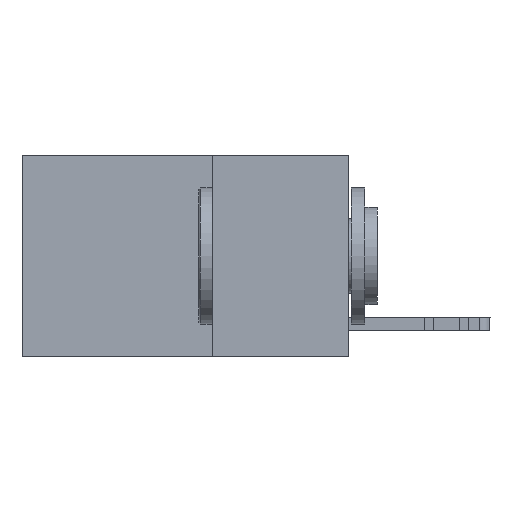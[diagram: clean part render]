
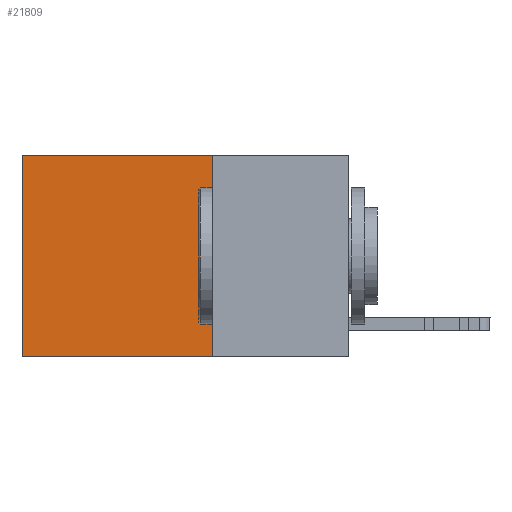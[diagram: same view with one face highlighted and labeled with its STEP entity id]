
A CAD part, left-side view. The second image highlights one B-rep face of the part: STEP entity #21809.
In plain terms, the highlighted planar face has unit normal (-1, 0, 0).
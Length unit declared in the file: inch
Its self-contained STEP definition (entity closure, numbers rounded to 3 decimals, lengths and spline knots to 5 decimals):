
#1019 = DIRECTION ( 'NONE',  ( 0., 0., -1. ) ) ;
#2023 = EDGE_CURVE ( 'NONE', #22591, #15932, #2679, .T. ) ;
#2591 = EDGE_CURVE ( 'NONE', #4354, #22591, #20277, .T. ) ;
#2679 = LINE ( 'NONE', #14874, #13444 ) ;
#3174 = VECTOR ( 'NONE', #3883, 39.37008 ) ;
#3883 = DIRECTION ( 'NONE',  ( 0., 0., -1. ) ) ;
#4354 = VERTEX_POINT ( 'NONE', #9734 ) ;
#4726 = VERTEX_POINT ( 'NONE', #6269 ) ;
#5284 = EDGE_LOOP ( 'NONE', ( #14977, #21265, #13969, #20225 ) ) ;
#5648 = LINE ( 'NONE', #24084, #22027 ) ;
#6269 = CARTESIAN_POINT ( 'NONE',  ( 0.2625, 0.6, 0. ) ) ;
#6828 = VECTOR ( 'NONE', #1019, 39.37008 ) ;
#9526 = EDGE_CURVE ( 'NONE', #4354, #4726, #5648, .T. ) ;
#9734 = CARTESIAN_POINT ( 'NONE',  ( 0.2625, 0.25, 0. ) ) ;
#11703 = EDGE_CURVE ( 'NONE', #4726, #15932, #11883, .T. ) ;
#11883 = LINE ( 'NONE', #24521, #6828 ) ;
#11989 = DIRECTION ( 'NONE',  ( 0., 0., -1. ) ) ;
#12637 = CARTESIAN_POINT ( 'NONE',  ( 0.2625, 0.6, -0.37 ) ) ;
#13444 = VECTOR ( 'NONE', #27551, 39.37008 ) ;
#13969 = ORIENTED_EDGE ( 'NONE', *, *, #2591, .F. ) ;
#14044 = CARTESIAN_POINT ( 'NONE',  ( 0.2625, 0.25, 0. ) ) ;
#14874 = CARTESIAN_POINT ( 'NONE',  ( 0.2625, 0.25, -0.37 ) ) ;
#14977 = ORIENTED_EDGE ( 'NONE', *, *, #11703, .T. ) ;
#15932 = VERTEX_POINT ( 'NONE', #12637 ) ;
#16967 = FACE_OUTER_BOUND ( 'NONE', #5284, .T. ) ;
#19332 = AXIS2_PLACEMENT_3D ( 'NONE', #14044, #24750, #11989 ) ;
#20225 = ORIENTED_EDGE ( 'NONE', *, *, #9526, .T. ) ;
#20277 = LINE ( 'NONE', #25170, #3174 ) ;
#21265 = ORIENTED_EDGE ( 'NONE', *, *, #2023, .F. ) ;
#21809 = ADVANCED_FACE ( 'NONE', ( #16967 ), #22634, .F. ) ;
#22027 = VECTOR ( 'NONE', #26174, 39.37008 ) ;
#22591 = VERTEX_POINT ( 'NONE', #26501 ) ;
#22634 = PLANE ( 'NONE',  #19332 ) ;
#24084 = CARTESIAN_POINT ( 'NONE',  ( 0.2625, 0.25, 0. ) ) ;
#24521 = CARTESIAN_POINT ( 'NONE',  ( 0.2625, 0.6, 0. ) ) ;
#24750 = DIRECTION ( 'NONE',  ( 1., 0., 0. ) ) ;
#25170 = CARTESIAN_POINT ( 'NONE',  ( 0.2625, 0.25, 0. ) ) ;
#26174 = DIRECTION ( 'NONE',  ( 0., 1., 0. ) ) ;
#26501 = CARTESIAN_POINT ( 'NONE',  ( 0.2625, 0.25, -0.37 ) ) ;
#27551 = DIRECTION ( 'NONE',  ( 0., 1., 0. ) ) ;
